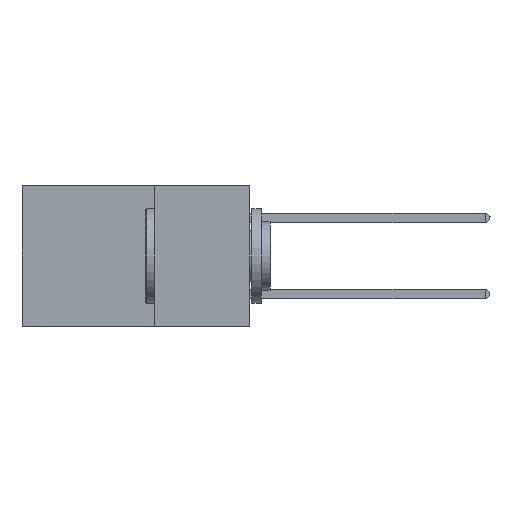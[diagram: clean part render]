
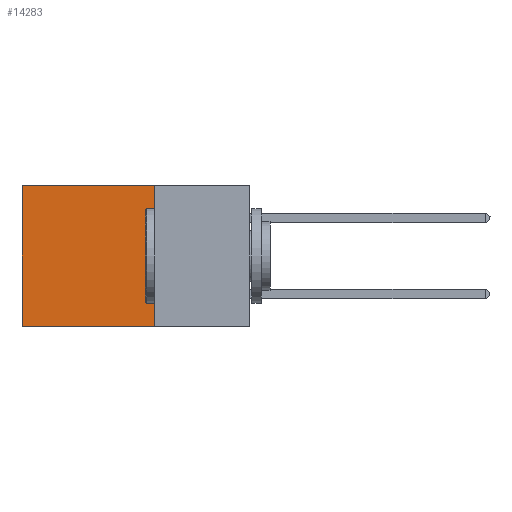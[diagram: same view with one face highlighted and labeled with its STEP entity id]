
A CAD part, left-side view. The second image highlights one B-rep face of the part: STEP entity #14283.
In plain terms, the highlighted planar face has unit normal (-1, 0, 0).
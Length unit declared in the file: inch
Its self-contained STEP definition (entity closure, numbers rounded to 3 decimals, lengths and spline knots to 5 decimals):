
#777 = VERTEX_POINT ( 'NONE', #15156 ) ;
#2433 = CARTESIAN_POINT ( 'NONE',  ( 0.2875, 0.25, 0. ) ) ;
#2810 = VERTEX_POINT ( 'NONE', #5329 ) ;
#4108 = LINE ( 'NONE', #2433, #12835 ) ;
#4117 = PLANE ( 'NONE',  #9829 ) ;
#4967 = ORIENTED_EDGE ( 'NONE', *, *, #14321, .F. ) ;
#5329 = CARTESIAN_POINT ( 'NONE',  ( 0.2875, 0.6, 0. ) ) ;
#5842 = CARTESIAN_POINT ( 'NONE',  ( 0.2875, 0.6, 0. ) ) ;
#5946 = EDGE_CURVE ( 'NONE', #2810, #18851, #22048, .T. ) ;
#6385 = VECTOR ( 'NONE', #16130, 39.37008 ) ;
#7628 = DIRECTION ( 'NONE',  ( 1., 0., 0. ) ) ;
#8656 = CARTESIAN_POINT ( 'NONE',  ( 0.2875, 0.6, -0.37 ) ) ;
#9329 = DIRECTION ( 'NONE',  ( 0., 1., 0. ) ) ;
#9829 = AXIS2_PLACEMENT_3D ( 'NONE', #11076, #7628, #19753 ) ;
#10533 = EDGE_LOOP ( 'NONE', ( #13009, #13249, #4967, #10947 ) ) ;
#10947 = ORIENTED_EDGE ( 'NONE', *, *, #20209, .T. ) ;
#11076 = CARTESIAN_POINT ( 'NONE',  ( 0.2875, 0.25, 0. ) ) ;
#12835 = VECTOR ( 'NONE', #16348, 39.37008 ) ;
#13009 = ORIENTED_EDGE ( 'NONE', *, *, #5946, .T. ) ;
#13249 = ORIENTED_EDGE ( 'NONE', *, *, #17925, .F. ) ;
#13661 = VERTEX_POINT ( 'NONE', #19836 ) ;
#14283 = ADVANCED_FACE ( 'NONE', ( #18470 ), #4117, .F. ) ;
#14321 = EDGE_CURVE ( 'NONE', #13661, #777, #4108, .T. ) ;
#14870 = VECTOR ( 'NONE', #9329, 39.37008 ) ;
#15156 = CARTESIAN_POINT ( 'NONE',  ( 0.2875, 0.25, -0.37 ) ) ;
#16130 = DIRECTION ( 'NONE',  ( 0., 1., 0. ) ) ;
#16209 = LINE ( 'NONE', #19582, #6385 ) ;
#16348 = DIRECTION ( 'NONE',  ( 0., 0., -1. ) ) ;
#16854 = VECTOR ( 'NONE', #19720, 39.37008 ) ;
#17925 = EDGE_CURVE ( 'NONE', #777, #18851, #16209, .T. ) ;
#17940 = CARTESIAN_POINT ( 'NONE',  ( 0.2875, 0.25, 0. ) ) ;
#18470 = FACE_OUTER_BOUND ( 'NONE', #10533, .T. ) ;
#18476 = LINE ( 'NONE', #17940, #14870 ) ;
#18851 = VERTEX_POINT ( 'NONE', #8656 ) ;
#19582 = CARTESIAN_POINT ( 'NONE',  ( 0.2875, 0.25, -0.37 ) ) ;
#19720 = DIRECTION ( 'NONE',  ( 0., 0., -1. ) ) ;
#19753 = DIRECTION ( 'NONE',  ( 0., 0., -1. ) ) ;
#19836 = CARTESIAN_POINT ( 'NONE',  ( 0.2875, 0.25, 0. ) ) ;
#20209 = EDGE_CURVE ( 'NONE', #13661, #2810, #18476, .T. ) ;
#22048 = LINE ( 'NONE', #5842, #16854 ) ;
